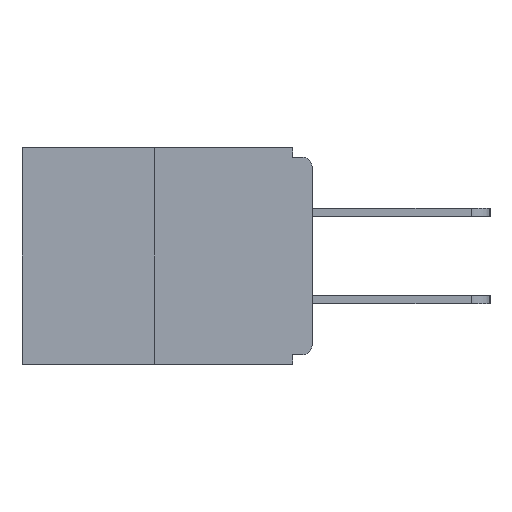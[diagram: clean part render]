
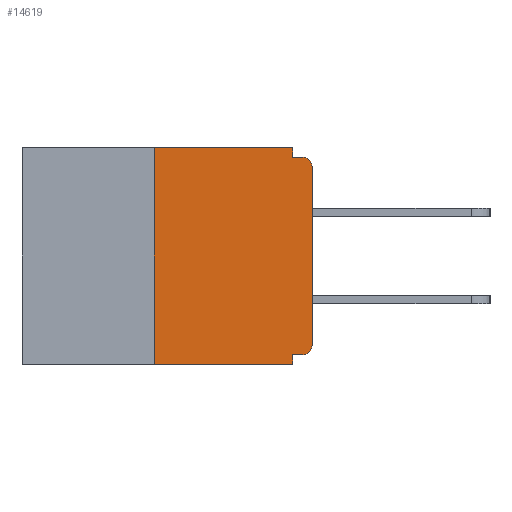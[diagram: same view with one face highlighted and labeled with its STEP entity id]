
A CAD part, left-side view. The second image highlights one B-rep face of the part: STEP entity #14619.
In plain terms, the highlighted planar face has unit normal (-1, 0, 0).
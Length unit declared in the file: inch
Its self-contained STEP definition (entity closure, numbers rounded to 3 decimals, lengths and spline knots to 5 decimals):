
#45 = ORIENTED_EDGE ( 'NONE', *, *, #9064, .F. ) ;
#273 = AXIS2_PLACEMENT_3D ( 'NONE', #17410, #28227, #8553 ) ;
#493 = LINE ( 'NONE', #2250, #7698 ) ;
#1203 = CARTESIAN_POINT ( 'NONE',  ( 0., 0.015, -0.015 ) ) ;
#1546 = CARTESIAN_POINT ( 'NONE',  ( 0., 0.015, -0.313 ) ) ;
#1577 = CARTESIAN_POINT ( 'NONE',  ( 0., 0., -0.015 ) ) ;
#1956 = CARTESIAN_POINT ( 'NONE',  ( 0., 0., -0.03 ) ) ;
#2250 = CARTESIAN_POINT ( 'NONE',  ( 0., 0., -0.328 ) ) ;
#2271 = LINE ( 'NONE', #21114, #19419 ) ;
#2625 = CARTESIAN_POINT ( 'NONE',  ( 0., 0.46, 0. ) ) ;
#2932 = LINE ( 'NONE', #23351, #14171 ) ;
#2973 = FACE_OUTER_BOUND ( 'NONE', #18622, .T. ) ;
#3700 = ORIENTED_EDGE ( 'NONE', *, *, #19407, .F. ) ;
#4017 = CARTESIAN_POINT ( 'NONE',  ( 0., 0.031, -0.328 ) ) ;
#4717 = VECTOR ( 'NONE', #22148, 39.37008 ) ;
#5103 = ORIENTED_EDGE ( 'NONE', *, *, #15755, .F. ) ;
#5463 = ORIENTED_EDGE ( 'NONE', *, *, #22455, .F. ) ;
#5487 = DIRECTION ( 'NONE',  ( 0., 0., -1. ) ) ;
#6117 = CIRCLE ( 'NONE', #273, 0.015 ) ;
#6296 = EDGE_CURVE ( 'NONE', #18418, #26253, #2271, .T. ) ;
#6514 = VERTEX_POINT ( 'NONE', #15229 ) ;
#7121 = VERTEX_POINT ( 'NONE', #25098 ) ;
#7180 = EDGE_CURVE ( 'NONE', #18418, #26224, #2932, .T. ) ;
#7330 = CARTESIAN_POINT ( 'NONE',  ( 0., 0., 0. ) ) ;
#7392 = CARTESIAN_POINT ( 'NONE',  ( 0., 0.25, -0.343 ) ) ;
#7441 = EDGE_CURVE ( 'NONE', #22774, #7121, #21758, .T. ) ;
#7511 = DIRECTION ( 'NONE',  ( 1., 0., 0. ) ) ;
#7698 = VECTOR ( 'NONE', #10941, 39.37008 ) ;
#8369 = DIRECTION ( 'NONE',  ( 0., -1., 0. ) ) ;
#8553 = DIRECTION ( 'NONE',  ( 0., 0., -1. ) ) ;
#8757 = VERTEX_POINT ( 'NONE', #1203 ) ;
#9064 = EDGE_CURVE ( 'NONE', #26224, #6514, #9974, .T. ) ;
#9159 = LINE ( 'NONE', #26503, #4717 ) ;
#9974 = LINE ( 'NONE', #2625, #22330 ) ;
#9984 = PLANE ( 'NONE',  #24467 ) ;
#10030 = CARTESIAN_POINT ( 'NONE',  ( 0., 0.031, 0. ) ) ;
#10184 = DIRECTION ( 'NONE',  ( 0., 0., 1. ) ) ;
#10941 = DIRECTION ( 'NONE',  ( 0., 1., 0. ) ) ;
#11644 = EDGE_CURVE ( 'NONE', #7121, #27764, #22558, .T. ) ;
#12145 = DIRECTION ( 'NONE',  ( -1., 0., 0. ) ) ;
#12209 = DIRECTION ( 'NONE',  ( 0., 0., -1. ) ) ;
#12458 = VECTOR ( 'NONE', #12209, 39.37008 ) ;
#12518 = CARTESIAN_POINT ( 'NONE',  ( 0., 0.031, -0.343 ) ) ;
#13159 = EDGE_CURVE ( 'NONE', #24771, #26253, #9159, .T. ) ;
#13608 = VERTEX_POINT ( 'NONE', #28185 ) ;
#13988 = ORIENTED_EDGE ( 'NONE', *, *, #7180, .F. ) ;
#14034 = VECTOR ( 'NONE', #8369, 39.37008 ) ;
#14125 = ORIENTED_EDGE ( 'NONE', *, *, #11644, .T. ) ;
#14163 = AXIS2_PLACEMENT_3D ( 'NONE', #1546, #12145, #27916 ) ;
#14171 = VECTOR ( 'NONE', #10184, 39.37008 ) ;
#14619 = ADVANCED_FACE ( 'NONE', ( #2973 ), #9984, .F. ) ;
#14626 = VECTOR ( 'NONE', #24872, 39.37008 ) ;
#15229 = CARTESIAN_POINT ( 'NONE',  ( 0., 0.031, 0. ) ) ;
#15755 = EDGE_CURVE ( 'NONE', #22774, #24771, #493, .T. ) ;
#16375 = ORIENTED_EDGE ( 'NONE', *, *, #7441, .T. ) ;
#16917 = LINE ( 'NONE', #10030, #12458 ) ;
#17410 = CARTESIAN_POINT ( 'NONE',  ( 0., 0.015, -0.03 ) ) ;
#17967 = ORIENTED_EDGE ( 'NONE', *, *, #25300, .T. ) ;
#18418 = VERTEX_POINT ( 'NONE', #7392 ) ;
#18606 = CARTESIAN_POINT ( 'NONE',  ( 0., 0.46, 0. ) ) ;
#18622 = EDGE_LOOP ( 'NONE', ( #45, #13988, #25859, #27625, #5103, #16375, #14125, #17967, #5463, #3700 ) ) ;
#19407 = EDGE_CURVE ( 'NONE', #6514, #13608, #16917, .T. ) ;
#19419 = VECTOR ( 'NONE', #20740, 39.37008 ) ;
#20140 = DIRECTION ( 'NONE',  ( 0., -1., 0. ) ) ;
#20740 = DIRECTION ( 'NONE',  ( 0., -1., 0. ) ) ;
#20857 = CARTESIAN_POINT ( 'NONE',  ( 0., 0.015, -0.328 ) ) ;
#21114 = CARTESIAN_POINT ( 'NONE',  ( 0., 0.46, -0.343 ) ) ;
#21758 = CIRCLE ( 'NONE', #14163, 0.015 ) ;
#22148 = DIRECTION ( 'NONE',  ( 0., 0., -1. ) ) ;
#22330 = VECTOR ( 'NONE', #20140, 39.37008 ) ;
#22455 = EDGE_CURVE ( 'NONE', #13608, #8757, #23701, .T. ) ;
#22558 = LINE ( 'NONE', #7330, #14626 ) ;
#22774 = VERTEX_POINT ( 'NONE', #20857 ) ;
#23351 = CARTESIAN_POINT ( 'NONE',  ( 0., 0.25, 0. ) ) ;
#23701 = LINE ( 'NONE', #1577, #14034 ) ;
#24467 = AXIS2_PLACEMENT_3D ( 'NONE', #18606, #7511, #5487 ) ;
#24771 = VERTEX_POINT ( 'NONE', #4017 ) ;
#24872 = DIRECTION ( 'NONE',  ( 0., 0., 1. ) ) ;
#25098 = CARTESIAN_POINT ( 'NONE',  ( 0., 0., -0.313 ) ) ;
#25300 = EDGE_CURVE ( 'NONE', #27764, #8757, #6117, .T. ) ;
#25859 = ORIENTED_EDGE ( 'NONE', *, *, #6296, .T. ) ;
#26224 = VERTEX_POINT ( 'NONE', #27641 ) ;
#26253 = VERTEX_POINT ( 'NONE', #12518 ) ;
#26503 = CARTESIAN_POINT ( 'NONE',  ( 0., 0.031, -0.343 ) ) ;
#27625 = ORIENTED_EDGE ( 'NONE', *, *, #13159, .F. ) ;
#27641 = CARTESIAN_POINT ( 'NONE',  ( 0., 0.25, 0. ) ) ;
#27764 = VERTEX_POINT ( 'NONE', #1956 ) ;
#27916 = DIRECTION ( 'NONE',  ( 0., 0., -1. ) ) ;
#28185 = CARTESIAN_POINT ( 'NONE',  ( 0., 0.031, -0.015 ) ) ;
#28227 = DIRECTION ( 'NONE',  ( -1., 0., 0. ) ) ;
